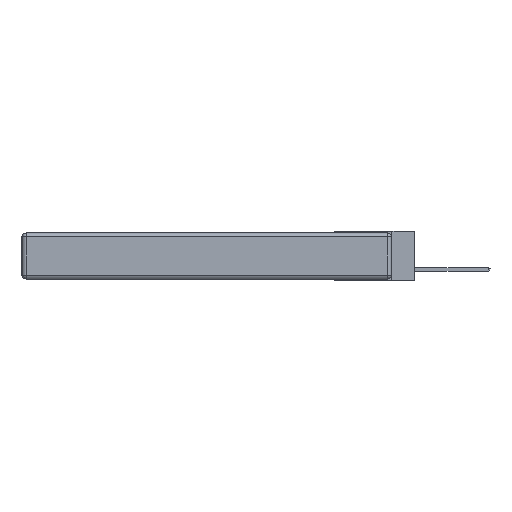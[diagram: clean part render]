
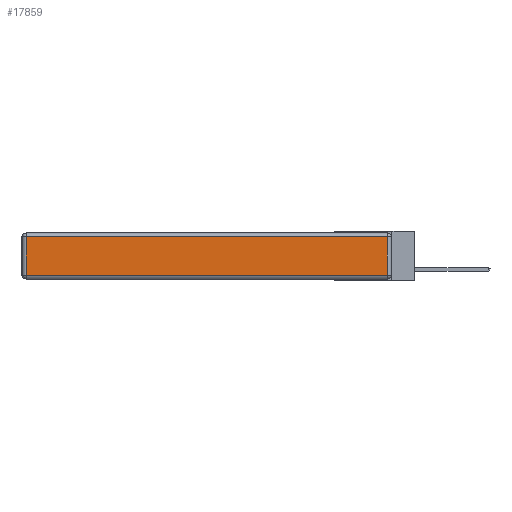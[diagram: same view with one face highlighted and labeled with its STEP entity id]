
A CAD part, left-side view. The second image highlights one B-rep face of the part: STEP entity #17859.
In plain terms, the highlighted planar face has unit normal (-1, 0, 0).
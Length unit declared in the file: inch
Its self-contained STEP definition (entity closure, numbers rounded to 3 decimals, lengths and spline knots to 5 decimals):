
#66 = VERTEX_POINT ( 'NONE', #13597 ) ;
#387 = VERTEX_POINT ( 'NONE', #25619 ) ;
#1135 = ORIENTED_EDGE ( 'NONE', *, *, #15176, .T. ) ;
#1481 = CARTESIAN_POINT ( 'NONE',  ( 0., 0., -0.313 ) ) ;
#1565 = DIRECTION ( 'NONE',  ( 0., 1., 0. ) ) ;
#3006 = LINE ( 'NONE', #24650, #5977 ) ;
#3617 = VECTOR ( 'NONE', #16225, 39.37008 ) ;
#5604 = VERTEX_POINT ( 'NONE', #16706 ) ;
#5791 = VECTOR ( 'NONE', #9792, 39.37008 ) ;
#5977 = VECTOR ( 'NONE', #1565, 39.37008 ) ;
#6160 = DIRECTION ( 'NONE',  ( -1., 0., 0. ) ) ;
#9792 = DIRECTION ( 'NONE',  ( 0., 0., -1. ) ) ;
#10816 = FACE_OUTER_BOUND ( 'NONE', #18985, .T. ) ;
#10948 = LINE ( 'NONE', #1481, #19248 ) ;
#12569 = ORIENTED_EDGE ( 'NONE', *, *, #15220, .T. ) ;
#13597 = CARTESIAN_POINT ( 'NONE',  ( 0., 0.03, -0.03 ) ) ;
#14165 = DIRECTION ( 'NONE',  ( 0., -1., 0. ) ) ;
#14623 = CARTESIAN_POINT ( 'NONE',  ( 0., 0., -0.343 ) ) ;
#14773 = VERTEX_POINT ( 'NONE', #27316 ) ;
#15176 = EDGE_CURVE ( 'NONE', #5604, #14773, #10948, .T. ) ;
#15220 = EDGE_CURVE ( 'NONE', #66, #387, #3006, .T. ) ;
#15570 = LINE ( 'NONE', #26710, #3617 ) ;
#16225 = DIRECTION ( 'NONE',  ( 0., 0., 1. ) ) ;
#16417 = LINE ( 'NONE', #24495, #5791 ) ;
#16706 = CARTESIAN_POINT ( 'NONE',  ( 0., 2.72, -0.313 ) ) ;
#17859 = ADVANCED_FACE ( 'NONE', ( #10816 ), #27043, .T. ) ;
#18695 = DIRECTION ( 'NONE',  ( 0., 0., 1. ) ) ;
#18985 = EDGE_LOOP ( 'NONE', ( #1135, #19951, #12569, #21969 ) ) ;
#19248 = VECTOR ( 'NONE', #14165, 39.37008 ) ;
#19754 = AXIS2_PLACEMENT_3D ( 'NONE', #14623, #6160, #18695 ) ;
#19951 = ORIENTED_EDGE ( 'NONE', *, *, #23678, .T. ) ;
#20940 = EDGE_CURVE ( 'NONE', #387, #5604, #16417, .T. ) ;
#21969 = ORIENTED_EDGE ( 'NONE', *, *, #20940, .T. ) ;
#23678 = EDGE_CURVE ( 'NONE', #14773, #66, #15570, .T. ) ;
#24495 = CARTESIAN_POINT ( 'NONE',  ( 0., 2.72, -0.343 ) ) ;
#24650 = CARTESIAN_POINT ( 'NONE',  ( 0., 2.75, -0.03 ) ) ;
#25619 = CARTESIAN_POINT ( 'NONE',  ( 0., 2.72, -0.03 ) ) ;
#26710 = CARTESIAN_POINT ( 'NONE',  ( 0., 0.03, -0.343 ) ) ;
#27043 = PLANE ( 'NONE',  #19754 ) ;
#27316 = CARTESIAN_POINT ( 'NONE',  ( 0., 0.03, -0.313 ) ) ;
